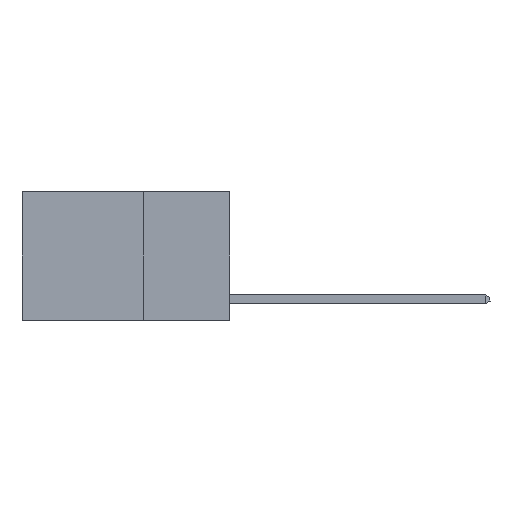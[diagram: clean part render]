
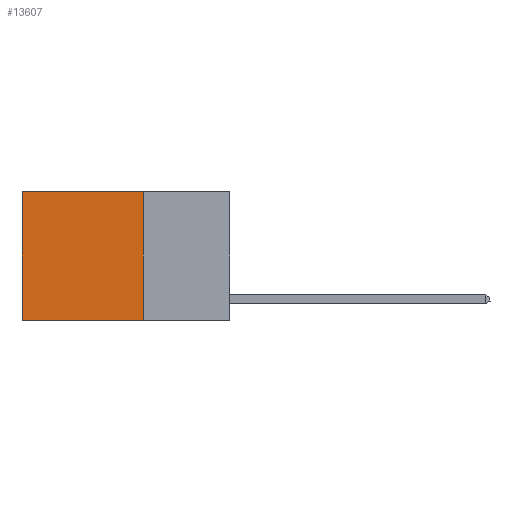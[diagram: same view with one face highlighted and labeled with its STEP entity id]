
A CAD part, left-side view. The second image highlights one B-rep face of the part: STEP entity #13607.
In plain terms, the highlighted planar face has unit normal (-1, 0, 0).
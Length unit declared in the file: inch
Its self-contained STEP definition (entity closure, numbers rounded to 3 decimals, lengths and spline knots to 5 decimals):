
#11 = DIRECTION ( 'NONE',  ( 1., 0., 0. ) ) ;
#46 = ORIENTED_EDGE ( 'NONE', *, *, #4016, .T. ) ;
#184 = EDGE_CURVE ( 'NONE', #13840, #8091, #6768, .T. ) ;
#661 = ORIENTED_EDGE ( 'NONE', *, *, #5365, .F. ) ;
#729 = CARTESIAN_POINT ( 'NONE',  ( 0.2625, 0.25, -0.37 ) ) ;
#1067 = DIRECTION ( 'NONE',  ( 0., 1., 0. ) ) ;
#1370 = LINE ( 'NONE', #8931, #13923 ) ;
#2136 = DIRECTION ( 'NONE',  ( 0., 0., -1. ) ) ;
#2255 = DIRECTION ( 'NONE',  ( 0., 0., -1. ) ) ;
#3061 = ORIENTED_EDGE ( 'NONE', *, *, #9574, .F. ) ;
#3791 = DIRECTION ( 'NONE',  ( 0., 1., 0. ) ) ;
#4016 = EDGE_CURVE ( 'NONE', #8091, #9062, #7969, .T. ) ;
#4390 = CARTESIAN_POINT ( 'NONE',  ( 0.2625, 0.6, 0. ) ) ;
#4819 = CARTESIAN_POINT ( 'NONE',  ( 0.2625, 0.6, -0.37 ) ) ;
#5365 = EDGE_CURVE ( 'NONE', #13840, #9946, #1370, .T. ) ;
#6311 = VECTOR ( 'NONE', #3791, 39.37008 ) ;
#6768 = LINE ( 'NONE', #11387, #7828 ) ;
#6824 = CARTESIAN_POINT ( 'NONE',  ( 0.2625, 0.25, 0. ) ) ;
#6905 = CARTESIAN_POINT ( 'NONE',  ( 0.2625, 0.6, 0. ) ) ;
#7828 = VECTOR ( 'NONE', #1067, 39.37008 ) ;
#7969 = LINE ( 'NONE', #4390, #12394 ) ;
#8091 = VERTEX_POINT ( 'NONE', #6905 ) ;
#8931 = CARTESIAN_POINT ( 'NONE',  ( 0.2625, 0.25, 0. ) ) ;
#9042 = PLANE ( 'NONE',  #9343 ) ;
#9062 = VERTEX_POINT ( 'NONE', #4819 ) ;
#9222 = FACE_OUTER_BOUND ( 'NONE', #13944, .T. ) ;
#9343 = AXIS2_PLACEMENT_3D ( 'NONE', #6824, #11, #2255 ) ;
#9574 = EDGE_CURVE ( 'NONE', #9946, #9062, #14585, .T. ) ;
#9946 = VERTEX_POINT ( 'NONE', #729 ) ;
#11387 = CARTESIAN_POINT ( 'NONE',  ( 0.2625, 0.25, 0. ) ) ;
#11710 = CARTESIAN_POINT ( 'NONE',  ( 0.2625, 0.25, -0.37 ) ) ;
#12394 = VECTOR ( 'NONE', #12479, 39.37008 ) ;
#12479 = DIRECTION ( 'NONE',  ( 0., 0., -1. ) ) ;
#12916 = ORIENTED_EDGE ( 'NONE', *, *, #184, .T. ) ;
#13607 = ADVANCED_FACE ( 'NONE', ( #9222 ), #9042, .F. ) ;
#13840 = VERTEX_POINT ( 'NONE', #14335 ) ;
#13923 = VECTOR ( 'NONE', #2136, 39.37008 ) ;
#13944 = EDGE_LOOP ( 'NONE', ( #46, #3061, #661, #12916 ) ) ;
#14335 = CARTESIAN_POINT ( 'NONE',  ( 0.2625, 0.25, 0. ) ) ;
#14585 = LINE ( 'NONE', #11710, #6311 ) ;
